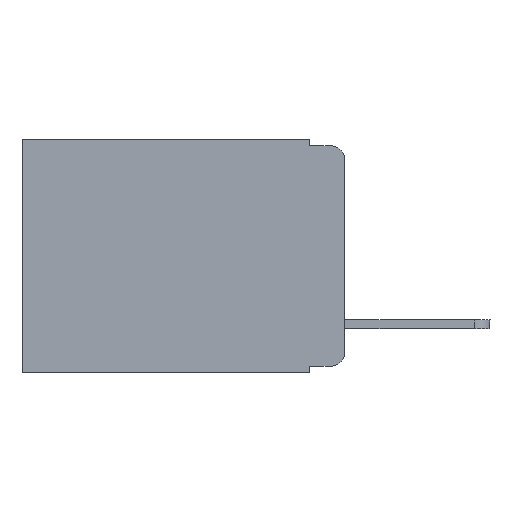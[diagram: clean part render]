
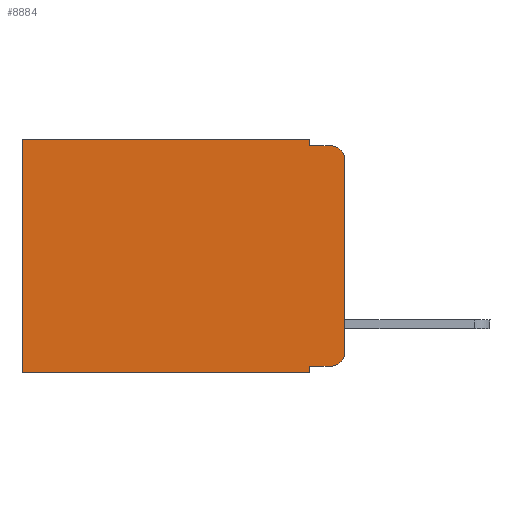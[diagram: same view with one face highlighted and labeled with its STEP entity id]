
A CAD part, left-side view. The second image highlights one B-rep face of the part: STEP entity #8884.
In plain terms, the highlighted planar face has unit normal (-1, 0, 0).
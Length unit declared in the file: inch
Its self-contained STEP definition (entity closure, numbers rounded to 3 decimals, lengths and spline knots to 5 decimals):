
#17 = VECTOR ( 'NONE', #13680, 39.37008 ) ;
#52 = EDGE_LOOP ( 'NONE', ( #3149, #6559, #1271, #18013, #7353, #12448, #1536, #11535, #11775, #5778 ) ) ;
#124 = EDGE_CURVE ( 'NONE', #12954, #11943, #7184, .T. ) ;
#833 = CARTESIAN_POINT ( 'NONE',  ( 0.298, 0.051, -0.333 ) ) ;
#860 = LINE ( 'NONE', #7045, #2604 ) ;
#1115 = LINE ( 'NONE', #7723, #3576 ) ;
#1271 = ORIENTED_EDGE ( 'NONE', *, *, #7042, .F. ) ;
#1488 = CARTESIAN_POINT ( 'NONE',  ( 0.298, 0., 0. ) ) ;
#1536 = ORIENTED_EDGE ( 'NONE', *, *, #11836, .F. ) ;
#1732 = VECTOR ( 'NONE', #9860, 39.37008 ) ;
#2022 = VECTOR ( 'NONE', #14452, 39.37008 ) ;
#2089 = DIRECTION ( 'NONE',  ( -1., 0., 0. ) ) ;
#2604 = VECTOR ( 'NONE', #12864, 39.37008 ) ;
#3138 = LINE ( 'NONE', #4584, #1732 ) ;
#3149 = ORIENTED_EDGE ( 'NONE', *, *, #124, .F. ) ;
#3576 = VECTOR ( 'NONE', #12567, 39.37008 ) ;
#3795 = VERTEX_POINT ( 'NONE', #15787 ) ;
#4016 = CARTESIAN_POINT ( 'NONE',  ( 0.298, 0.473, 0. ) ) ;
#4342 = EDGE_CURVE ( 'NONE', #7511, #11943, #8221, .T. ) ;
#4413 = CARTESIAN_POINT ( 'NONE',  ( 0.298, 0.051, 0. ) ) ;
#4584 = CARTESIAN_POINT ( 'NONE',  ( 0.298, 0., -0.343 ) ) ;
#4888 = CARTESIAN_POINT ( 'NONE',  ( 0.298, 0.051, 0. ) ) ;
#5486 = VECTOR ( 'NONE', #17755, 39.37008 ) ;
#5497 = CARTESIAN_POINT ( 'NONE',  ( 0.298, 0.02, -0.313 ) ) ;
#5660 = CIRCLE ( 'NONE', #11136, 0.02 ) ;
#5771 = EDGE_CURVE ( 'NONE', #9255, #7511, #8037, .T. ) ;
#5778 = ORIENTED_EDGE ( 'NONE', *, *, #4342, .T. ) ;
#6509 = CARTESIAN_POINT ( 'NONE',  ( 0.298, 0.051, -0.333 ) ) ;
#6559 = ORIENTED_EDGE ( 'NONE', *, *, #8816, .T. ) ;
#7042 = EDGE_CURVE ( 'NONE', #16445, #10898, #13266, .T. ) ;
#7045 = CARTESIAN_POINT ( 'NONE',  ( 0.298, 0.051, 0. ) ) ;
#7158 = CARTESIAN_POINT ( 'NONE',  ( 0.298, 0.051, -0.01 ) ) ;
#7184 = LINE ( 'NONE', #7286, #10094 ) ;
#7286 = CARTESIAN_POINT ( 'NONE',  ( 0.298, 0., 0. ) ) ;
#7353 = ORIENTED_EDGE ( 'NONE', *, *, #15379, .T. ) ;
#7377 = VERTEX_POINT ( 'NONE', #9746 ) ;
#7511 = VERTEX_POINT ( 'NONE', #15138 ) ;
#7723 = CARTESIAN_POINT ( 'NONE',  ( 0.298, 0.473, 0. ) ) ;
#7913 = DIRECTION ( 'NONE',  ( 0., 0., -1. ) ) ;
#8037 = LINE ( 'NONE', #6509, #17 ) ;
#8221 = CIRCLE ( 'NONE', #11283, 0.02 ) ;
#8321 = VERTEX_POINT ( 'NONE', #4888 ) ;
#8380 = PLANE ( 'NONE',  #8689 ) ;
#8442 = DIRECTION ( 'NONE',  ( -1., 0., 0. ) ) ;
#8626 = DIRECTION ( 'NONE',  ( 0., 0., -1. ) ) ;
#8689 = AXIS2_PLACEMENT_3D ( 'NONE', #9725, #11067, #14189 ) ;
#8816 = EDGE_CURVE ( 'NONE', #12954, #10898, #5660, .T. ) ;
#8884 = ADVANCED_FACE ( 'NONE', ( #15409 ), #8380, .F. ) ;
#8917 = EDGE_CURVE ( 'NONE', #8321, #16445, #860, .T. ) ;
#9255 = VERTEX_POINT ( 'NONE', #833 ) ;
#9336 = CARTESIAN_POINT ( 'NONE',  ( 0.298, 0.02, -0.03 ) ) ;
#9725 = CARTESIAN_POINT ( 'NONE',  ( 0.298, 0., 0. ) ) ;
#9746 = CARTESIAN_POINT ( 'NONE',  ( 0.298, 0.473, -0.343 ) ) ;
#9860 = DIRECTION ( 'NONE',  ( 0., 1., 0. ) ) ;
#10094 = VECTOR ( 'NONE', #8626, 39.37008 ) ;
#10898 = VERTEX_POINT ( 'NONE', #11140 ) ;
#11067 = DIRECTION ( 'NONE',  ( 1., 0., 0. ) ) ;
#11136 = AXIS2_PLACEMENT_3D ( 'NONE', #9336, #2089, #7913 ) ;
#11140 = CARTESIAN_POINT ( 'NONE',  ( 0.298, 0.02, -0.01 ) ) ;
#11283 = AXIS2_PLACEMENT_3D ( 'NONE', #5497, #8442, #14259 ) ;
#11535 = ORIENTED_EDGE ( 'NONE', *, *, #18316, .F. ) ;
#11717 = CARTESIAN_POINT ( 'NONE',  ( 0.298, 0., -0.313 ) ) ;
#11775 = ORIENTED_EDGE ( 'NONE', *, *, #5771, .T. ) ;
#11836 = EDGE_CURVE ( 'NONE', #3795, #7377, #3138, .T. ) ;
#11943 = VERTEX_POINT ( 'NONE', #11717 ) ;
#12448 = ORIENTED_EDGE ( 'NONE', *, *, #13810, .T. ) ;
#12567 = DIRECTION ( 'NONE',  ( 0., 0., -1. ) ) ;
#12864 = DIRECTION ( 'NONE',  ( 0., 0., -1. ) ) ;
#12954 = VERTEX_POINT ( 'NONE', #16799 ) ;
#13210 = LINE ( 'NONE', #1488, #2022 ) ;
#13266 = LINE ( 'NONE', #7158, #14959 ) ;
#13680 = DIRECTION ( 'NONE',  ( 0., -1., 0. ) ) ;
#13810 = EDGE_CURVE ( 'NONE', #17757, #7377, #1115, .T. ) ;
#14189 = DIRECTION ( 'NONE',  ( 0., 0., -1. ) ) ;
#14259 = DIRECTION ( 'NONE',  ( 0., 0., -1. ) ) ;
#14452 = DIRECTION ( 'NONE',  ( 0., 1., 0. ) ) ;
#14609 = DIRECTION ( 'NONE',  ( 0., -1., 0. ) ) ;
#14959 = VECTOR ( 'NONE', #14609, 39.37008 ) ;
#15138 = CARTESIAN_POINT ( 'NONE',  ( 0.298, 0.02, -0.333 ) ) ;
#15379 = EDGE_CURVE ( 'NONE', #8321, #17757, #13210, .T. ) ;
#15409 = FACE_OUTER_BOUND ( 'NONE', #52, .T. ) ;
#15787 = CARTESIAN_POINT ( 'NONE',  ( 0.298, 0.051, -0.343 ) ) ;
#16148 = LINE ( 'NONE', #4413, #5486 ) ;
#16445 = VERTEX_POINT ( 'NONE', #16556 ) ;
#16556 = CARTESIAN_POINT ( 'NONE',  ( 0.298, 0.051, -0.01 ) ) ;
#16799 = CARTESIAN_POINT ( 'NONE',  ( 0.298, 0., -0.03 ) ) ;
#17755 = DIRECTION ( 'NONE',  ( 0., 0., -1. ) ) ;
#17757 = VERTEX_POINT ( 'NONE', #4016 ) ;
#18013 = ORIENTED_EDGE ( 'NONE', *, *, #8917, .F. ) ;
#18316 = EDGE_CURVE ( 'NONE', #9255, #3795, #16148, .T. ) ;
